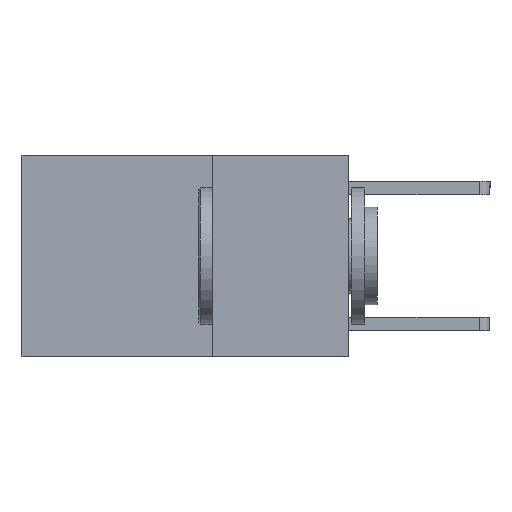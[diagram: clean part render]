
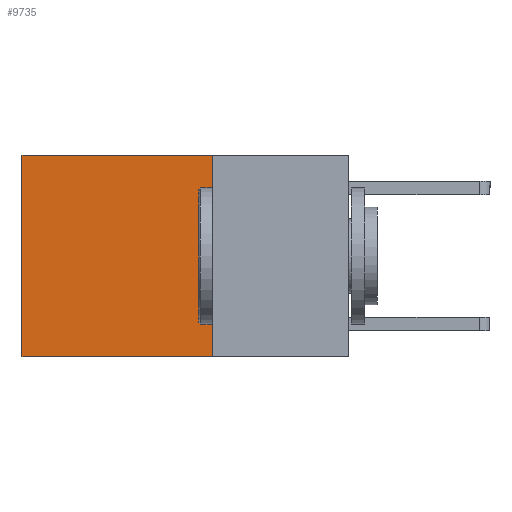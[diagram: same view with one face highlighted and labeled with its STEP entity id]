
A CAD part, left-side view. The second image highlights one B-rep face of the part: STEP entity #9735.
In plain terms, the highlighted planar face has unit normal (-1, 0, 0).
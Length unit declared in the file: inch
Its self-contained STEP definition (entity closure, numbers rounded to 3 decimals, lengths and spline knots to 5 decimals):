
#88 = DIRECTION ( 'NONE',  ( 0., 0., -1. ) ) ;
#312 = EDGE_CURVE ( 'NONE', #691, #2728, #6549, .T. ) ;
#691 = VERTEX_POINT ( 'NONE', #7824 ) ;
#931 = EDGE_CURVE ( 'NONE', #3343, #691, #4061, .T. ) ;
#1553 = CARTESIAN_POINT ( 'NONE',  ( 0.2625, 0.25, 0. ) ) ;
#2433 = ORIENTED_EDGE ( 'NONE', *, *, #4402, .T. ) ;
#2507 = CARTESIAN_POINT ( 'NONE',  ( 0.2625, 0.6, -0.37 ) ) ;
#2629 = CARTESIAN_POINT ( 'NONE',  ( 0.2625, 0.6, 0. ) ) ;
#2728 = VERTEX_POINT ( 'NONE', #2507 ) ;
#2879 = CARTESIAN_POINT ( 'NONE',  ( 0.2625, 0.25, 0. ) ) ;
#2932 = DIRECTION ( 'NONE',  ( 1., 0., 0. ) ) ;
#2935 = VECTOR ( 'NONE', #10538, 39.37008 ) ;
#3343 = VERTEX_POINT ( 'NONE', #4249 ) ;
#4061 = LINE ( 'NONE', #7496, #7023 ) ;
#4249 = CARTESIAN_POINT ( 'NONE',  ( 0.2625, 0.25, 0. ) ) ;
#4402 = EDGE_CURVE ( 'NONE', #3343, #8819, #5752, .T. ) ;
#4779 = VECTOR ( 'NONE', #88, 39.37008 ) ;
#4890 = ORIENTED_EDGE ( 'NONE', *, *, #312, .F. ) ;
#4920 = DIRECTION ( 'NONE',  ( 0., 1., 0. ) ) ;
#5304 = AXIS2_PLACEMENT_3D ( 'NONE', #2879, #2932, #10388 ) ;
#5730 = CARTESIAN_POINT ( 'NONE',  ( 0.2625, 0.25, -0.37 ) ) ;
#5752 = LINE ( 'NONE', #1553, #10662 ) ;
#5825 = DIRECTION ( 'NONE',  ( 0., 0., -1. ) ) ;
#5836 = EDGE_LOOP ( 'NONE', ( #9964, #4890, #8089, #2433 ) ) ;
#6549 = LINE ( 'NONE', #5730, #2935 ) ;
#7023 = VECTOR ( 'NONE', #5825, 39.37008 ) ;
#7138 = PLANE ( 'NONE',  #5304 ) ;
#7496 = CARTESIAN_POINT ( 'NONE',  ( 0.2625, 0.25, 0. ) ) ;
#7662 = LINE ( 'NONE', #2629, #4779 ) ;
#7824 = CARTESIAN_POINT ( 'NONE',  ( 0.2625, 0.25, -0.37 ) ) ;
#8089 = ORIENTED_EDGE ( 'NONE', *, *, #931, .F. ) ;
#8819 = VERTEX_POINT ( 'NONE', #9263 ) ;
#8901 = FACE_OUTER_BOUND ( 'NONE', #5836, .T. ) ;
#9112 = EDGE_CURVE ( 'NONE', #8819, #2728, #7662, .T. ) ;
#9263 = CARTESIAN_POINT ( 'NONE',  ( 0.2625, 0.6, 0. ) ) ;
#9735 = ADVANCED_FACE ( 'NONE', ( #8901 ), #7138, .F. ) ;
#9964 = ORIENTED_EDGE ( 'NONE', *, *, #9112, .T. ) ;
#10388 = DIRECTION ( 'NONE',  ( 0., 0., -1. ) ) ;
#10538 = DIRECTION ( 'NONE',  ( 0., 1., 0. ) ) ;
#10662 = VECTOR ( 'NONE', #4920, 39.37008 ) ;
